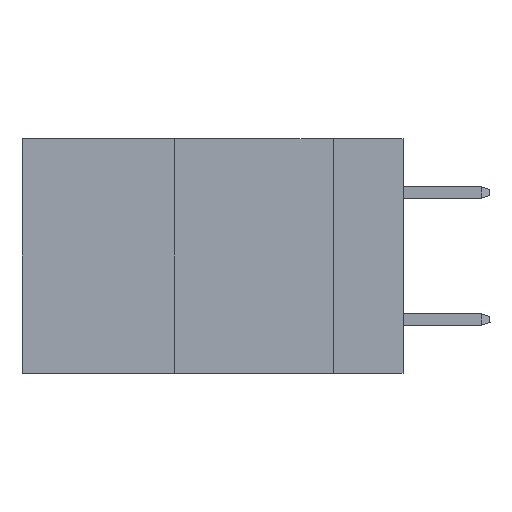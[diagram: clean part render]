
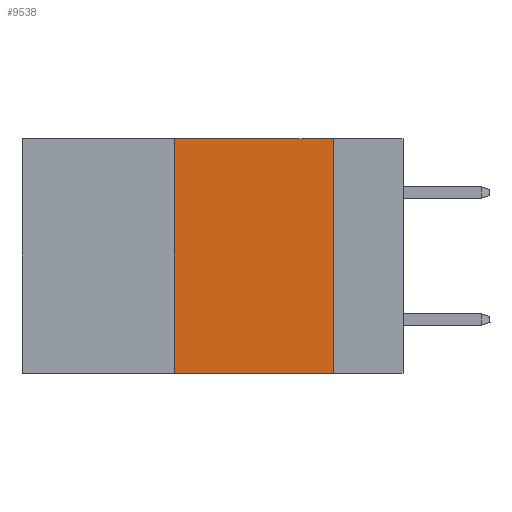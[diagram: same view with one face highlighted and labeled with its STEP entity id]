
A CAD part, left-side view. The second image highlights one B-rep face of the part: STEP entity #9538.
In plain terms, the highlighted planar face has unit normal (-1, 0, 0).
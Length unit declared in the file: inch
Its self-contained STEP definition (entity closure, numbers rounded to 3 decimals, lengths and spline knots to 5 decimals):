
#548 = DIRECTION ( 'NONE',  ( 0., 0., 1. ) ) ;
#699 = DIRECTION ( 'NONE',  ( 0., 0., -1. ) ) ;
#2166 = ORIENTED_EDGE ( 'NONE', *, *, #2537, .F. ) ;
#2455 = VECTOR ( 'NONE', #5907, 39.37008 ) ;
#2537 = EDGE_CURVE ( 'NONE', #13418, #4510, #5556, .T. ) ;
#2557 = VERTEX_POINT ( 'NONE', #3729 ) ;
#3443 = LINE ( 'NONE', #9914, #6336 ) ;
#3729 = CARTESIAN_POINT ( 'NONE',  ( 0., 0.11, 0. ) ) ;
#4020 = CARTESIAN_POINT ( 'NONE',  ( 0., 0.11, 0. ) ) ;
#4411 = DIRECTION ( 'NONE',  ( 0., -1., 0. ) ) ;
#4510 = VERTEX_POINT ( 'NONE', #10093 ) ;
#4615 = ORIENTED_EDGE ( 'NONE', *, *, #9915, .F. ) ;
#4638 = ORIENTED_EDGE ( 'NONE', *, *, #5165, .F. ) ;
#4972 = VECTOR ( 'NONE', #12886, 39.37008 ) ;
#5105 = LINE ( 'NONE', #4020, #4972 ) ;
#5165 = EDGE_CURVE ( 'NONE', #4510, #2557, #3443, .T. ) ;
#5556 = LINE ( 'NONE', #13882, #7195 ) ;
#5907 = DIRECTION ( 'NONE',  ( 0., -1., 0. ) ) ;
#6336 = VECTOR ( 'NONE', #4411, 39.37008 ) ;
#6364 = FACE_OUTER_BOUND ( 'NONE', #13853, .T. ) ;
#7195 = VECTOR ( 'NONE', #548, 39.37008 ) ;
#8076 = CARTESIAN_POINT ( 'NONE',  ( 0., 0.6, -0.37 ) ) ;
#8272 = ORIENTED_EDGE ( 'NONE', *, *, #11493, .T. ) ;
#8535 = CARTESIAN_POINT ( 'NONE',  ( 0., 0.6, 0. ) ) ;
#9538 = ADVANCED_FACE ( 'NONE', ( #6364 ), #9687, .F. ) ;
#9687 = PLANE ( 'NONE',  #13538 ) ;
#9915 = EDGE_CURVE ( 'NONE', #2557, #11344, #5105, .T. ) ;
#9914 = CARTESIAN_POINT ( 'NONE',  ( 0., 0.6, 0. ) ) ;
#10093 = CARTESIAN_POINT ( 'NONE',  ( 0., 0.36, 0. ) ) ;
#10642 = DIRECTION ( 'NONE',  ( 1., 0., 0. ) ) ;
#10989 = CARTESIAN_POINT ( 'NONE',  ( 0., 0.36, -0.37 ) ) ;
#11344 = VERTEX_POINT ( 'NONE', #13440 ) ;
#11493 = EDGE_CURVE ( 'NONE', #13418, #11344, #13510, .T. ) ;
#12886 = DIRECTION ( 'NONE',  ( 0., 0., -1. ) ) ;
#13418 = VERTEX_POINT ( 'NONE', #10989 ) ;
#13440 = CARTESIAN_POINT ( 'NONE',  ( 0., 0.11, -0.37 ) ) ;
#13510 = LINE ( 'NONE', #8076, #2455 ) ;
#13538 = AXIS2_PLACEMENT_3D ( 'NONE', #8535, #10642, #699 ) ;
#13853 = EDGE_LOOP ( 'NONE', ( #4615, #4638, #2166, #8272 ) ) ;
#13882 = CARTESIAN_POINT ( 'NONE',  ( 0., 0.36, 0. ) ) ;
